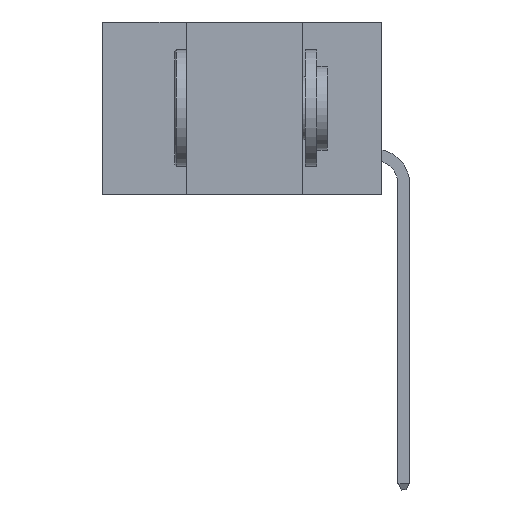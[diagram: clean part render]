
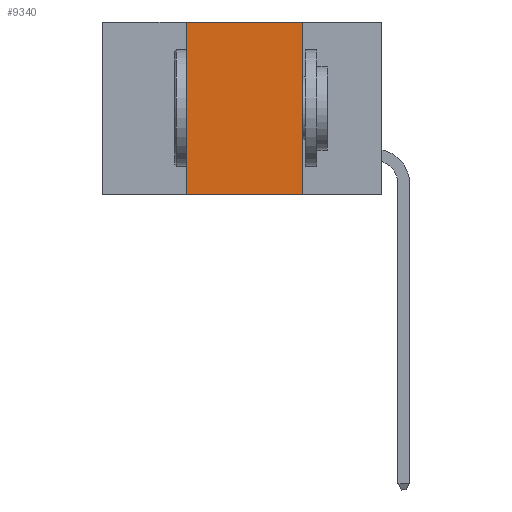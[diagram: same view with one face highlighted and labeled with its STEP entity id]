
A CAD part, left-side view. The second image highlights one B-rep face of the part: STEP entity #9340.
In plain terms, the highlighted planar face has unit normal (-1, 0, 0).
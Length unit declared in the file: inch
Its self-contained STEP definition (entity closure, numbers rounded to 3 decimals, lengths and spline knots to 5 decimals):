
#260 = EDGE_CURVE ( 'NONE', #16506, #7477, #11747, .T. ) ;
#502 = CARTESIAN_POINT ( 'NONE',  ( 0., 0.6, 0. ) ) ;
#585 = DIRECTION ( 'NONE',  ( 0., 0., -1. ) ) ;
#1045 = DIRECTION ( 'NONE',  ( 0., 0., -1. ) ) ;
#1125 = CARTESIAN_POINT ( 'NONE',  ( 0., 0.6, -0.37 ) ) ;
#2113 = DIRECTION ( 'NONE',  ( 0., -1., 0. ) ) ;
#2296 = EDGE_CURVE ( 'NONE', #7477, #7722, #4109, .T. ) ;
#2337 = VERTEX_POINT ( 'NONE', #16687 ) ;
#2905 = DIRECTION ( 'NONE',  ( 0., -1., 0. ) ) ;
#3564 = EDGE_LOOP ( 'NONE', ( #6889, #15566, #16533, #21103 ) ) ;
#4109 = LINE ( 'NONE', #502, #16304 ) ;
#4424 = CARTESIAN_POINT ( 'NONE',  ( 0., 0.42, 0. ) ) ;
#5928 = CARTESIAN_POINT ( 'NONE',  ( 0., 0.42, 0. ) ) ;
#6493 = DIRECTION ( 'NONE',  ( 0., 0., 1. ) ) ;
#6889 = ORIENTED_EDGE ( 'NONE', *, *, #19567, .F. ) ;
#7373 = VECTOR ( 'NONE', #6493, 39.37008 ) ;
#7477 = VERTEX_POINT ( 'NONE', #4424 ) ;
#7722 = VERTEX_POINT ( 'NONE', #10724 ) ;
#8340 = LINE ( 'NONE', #1125, #20021 ) ;
#9340 = ADVANCED_FACE ( 'NONE', ( #16471 ), #18811, .F. ) ;
#9935 = LINE ( 'NONE', #16168, #18367 ) ;
#10253 = AXIS2_PLACEMENT_3D ( 'NONE', #17263, #10921, #585 ) ;
#10724 = CARTESIAN_POINT ( 'NONE',  ( 0., 0.17, 0. ) ) ;
#10921 = DIRECTION ( 'NONE',  ( 1., 0., 0. ) ) ;
#11747 = LINE ( 'NONE', #5928, #7373 ) ;
#15566 = ORIENTED_EDGE ( 'NONE', *, *, #2296, .F. ) ;
#16168 = CARTESIAN_POINT ( 'NONE',  ( 0., 0.17, 0. ) ) ;
#16304 = VECTOR ( 'NONE', #2113, 39.37008 ) ;
#16471 = FACE_OUTER_BOUND ( 'NONE', #3564, .T. ) ;
#16506 = VERTEX_POINT ( 'NONE', #18740 ) ;
#16533 = ORIENTED_EDGE ( 'NONE', *, *, #260, .F. ) ;
#16687 = CARTESIAN_POINT ( 'NONE',  ( 0., 0.17, -0.37 ) ) ;
#17263 = CARTESIAN_POINT ( 'NONE',  ( 0., 0.6, 0. ) ) ;
#18367 = VECTOR ( 'NONE', #1045, 39.37008 ) ;
#18740 = CARTESIAN_POINT ( 'NONE',  ( 0., 0.42, -0.37 ) ) ;
#18811 = PLANE ( 'NONE',  #10253 ) ;
#19567 = EDGE_CURVE ( 'NONE', #7722, #2337, #9935, .T. ) ;
#20021 = VECTOR ( 'NONE', #2905, 39.37008 ) ;
#20590 = EDGE_CURVE ( 'NONE', #16506, #2337, #8340, .T. ) ;
#21103 = ORIENTED_EDGE ( 'NONE', *, *, #20590, .T. ) ;
